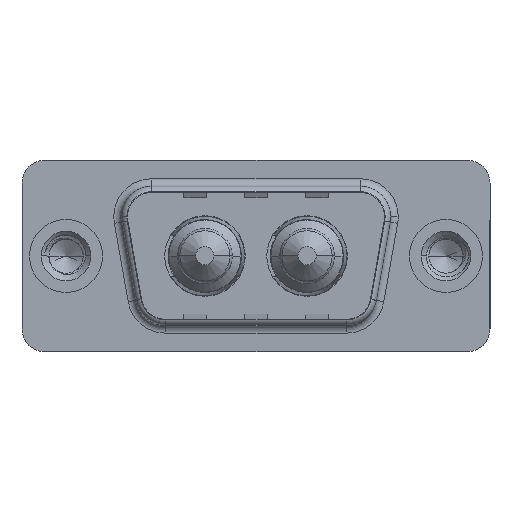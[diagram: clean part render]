
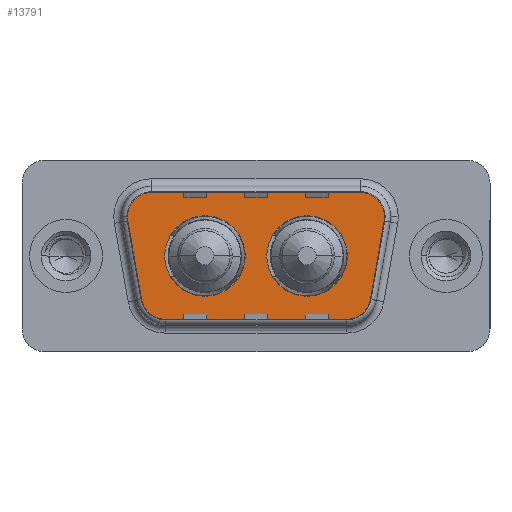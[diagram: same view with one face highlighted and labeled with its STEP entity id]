
A CAD part, top view. The second image highlights one B-rep face of the part: STEP entity #13791.
In plain terms, the highlighted planar face has unit normal (0, 0, 1).
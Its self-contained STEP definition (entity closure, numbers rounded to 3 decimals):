
#333 = DIRECTION ( 'NONE',  ( 1., 0., 0. ) ) ;
#508 = EDGE_CURVE ( 'NONE', #4184, #7738, #15613, .T. ) ;
#585 = EDGE_CURVE ( 'NONE', #8998, #4009, #1623, .T. ) ;
#634 = ORIENTED_EDGE ( 'NONE', *, *, #4315, .F. ) ;
#1050 = VERTEX_POINT ( 'NONE', #10100 ) ;
#1607 = CIRCLE ( 'NONE', #13384, 2. ) ;
#1623 = LINE ( 'NONE', #12045, #7820 ) ;
#1780 = EDGE_CURVE ( 'NONE', #1050, #6026, #15411, .T. ) ;
#2015 = VECTOR ( 'NONE', #2477, 1000. ) ;
#2201 = VECTOR ( 'NONE', #15428, 1000. ) ;
#2207 = EDGE_CURVE ( 'NONE', #7170, #6162, #10963, .T. ) ;
#2226 = EDGE_CURVE ( 'NONE', #14384, #4184, #1607, .T. ) ;
#2374 = CARTESIAN_POINT ( 'NONE',  ( 19.564, 2.9, 0. ) ) ;
#2419 = EDGE_CURVE ( 'NONE', #6162, #11359, #12398, .T. ) ;
#2477 = DIRECTION ( 'NONE',  ( -1., 0., 0. ) ) ;
#2572 = AXIS2_PLACEMENT_3D ( 'NONE', #5162, #15972, #12566 ) ;
#2642 = ORIENTED_EDGE ( 'NONE', *, *, #10940, .F. ) ;
#2664 = PLANE ( 'NONE',  #12718 ) ;
#2743 = CARTESIAN_POINT ( 'NONE',  ( 5.436, 4.9, 0. ) ) ;
#2938 = CARTESIAN_POINT ( 'NONE',  ( 5.436, 2.9, 0. ) ) ;
#3578 = CARTESIAN_POINT ( 'NONE',  ( 6.459, -4.9, 0. ) ) ;
#3645 = ORIENTED_EDGE ( 'NONE', *, *, #508, .T. ) ;
#3659 = DIRECTION ( 'NONE',  ( -1., 0., 0. ) ) ;
#3669 = AXIS2_PLACEMENT_3D ( 'NONE', #6401, #7185, #7149 ) ;
#3934 = DIRECTION ( 'NONE',  ( 1., 0., 0. ) ) ;
#3965 = VERTEX_POINT ( 'NONE', #11274 ) ;
#4009 = VERTEX_POINT ( 'NONE', #14877 ) ;
#4057 = CIRCLE ( 'NONE', #5607, 2. ) ;
#4184 = VERTEX_POINT ( 'NONE', #5513 ) ;
#4235 = DIRECTION ( 'NONE',  ( 1., 0., 0. ) ) ;
#4248 = AXIS2_PLACEMENT_3D ( 'NONE', #2374, #11283, #3659 ) ;
#4315 = EDGE_CURVE ( 'NONE', #15826, #9567, #7523, .T. ) ;
#4440 = CARTESIAN_POINT ( 'NONE',  ( 19.564, 2.9, 0. ) ) ;
#4667 = EDGE_CURVE ( 'NONE', #6026, #1050, #10710, .T. ) ;
#4704 = LINE ( 'NONE', #3578, #10680 ) ;
#4769 = ORIENTED_EDGE ( 'NONE', *, *, #2419, .T. ) ;
#4831 = CARTESIAN_POINT ( 'NONE',  ( 13.21, 0., 0. ) ) ;
#4928 = CARTESIAN_POINT ( 'NONE',  ( 3.466, 2.553, 0. ) ) ;
#4992 = DIRECTION ( 'NONE',  ( 0., 0., 1. ) ) ;
#5029 = CARTESIAN_POINT ( 'NONE',  ( 11.79, 0., 0. ) ) ;
#5162 = CARTESIAN_POINT ( 'NONE',  ( 15.86, 0., 0. ) ) ;
#5513 = CARTESIAN_POINT ( 'NONE',  ( 19.564, 4.9, 0. ) ) ;
#5607 = AXIS2_PLACEMENT_3D ( 'NONE', #12652, #4992, #13917 ) ;
#5917 = EDGE_CURVE ( 'NONE', #3965, #7170, #4704, .T. ) ;
#6026 = VERTEX_POINT ( 'NONE', #4831 ) ;
#6162 = VERTEX_POINT ( 'NONE', #15930 ) ;
#6401 = CARTESIAN_POINT ( 'NONE',  ( 15.86, 0., 0. ) ) ;
#6519 = DIRECTION ( 'NONE',  ( 1., 0., 0. ) ) ;
#6586 = ORIENTED_EDGE ( 'NONE', *, *, #8047, .T. ) ;
#7071 = DIRECTION ( 'NONE',  ( 0., 0., 1. ) ) ;
#7118 = EDGE_LOOP ( 'NONE', ( #2642, #634 ) ) ;
#7149 = DIRECTION ( 'NONE',  ( 1., 0., 0. ) ) ;
#7170 = VERTEX_POINT ( 'NONE', #13029 ) ;
#7185 = DIRECTION ( 'NONE',  ( 0., 0., 1. ) ) ;
#7472 = CARTESIAN_POINT ( 'NONE',  ( 5.436, 4.9, 0. ) ) ;
#7509 = EDGE_CURVE ( 'NONE', #4009, #3965, #4057, .T. ) ;
#7523 = CIRCLE ( 'NONE', #12857, 2.65 ) ;
#7738 = VERTEX_POINT ( 'NONE', #2743 ) ;
#7820 = VECTOR ( 'NONE', #11734, 1000. ) ;
#7966 = DIRECTION ( 'NONE',  ( 0., 0., 1. ) ) ;
#8047 = EDGE_CURVE ( 'NONE', #7738, #8998, #8244, .T. ) ;
#8189 = ORIENTED_EDGE ( 'NONE', *, *, #2226, .T. ) ;
#8205 = EDGE_LOOP ( 'NONE', ( #10204, #4769, #11759, #8189, #3645, #6586, #12038, #10561, #8634 ) ) ;
#8244 = CIRCLE ( 'NONE', #14396, 2. ) ;
#8346 = DIRECTION ( 'NONE',  ( 0., 0., 1. ) ) ;
#8549 = FACE_BOUND ( 'NONE', #7118, .T. ) ;
#8634 = ORIENTED_EDGE ( 'NONE', *, *, #5917, .T. ) ;
#8866 = AXIS2_PLACEMENT_3D ( 'NONE', #15650, #7966, #333 ) ;
#8954 = FACE_OUTER_BOUND ( 'NONE', #8205, .T. ) ;
#8998 = VERTEX_POINT ( 'NONE', #4928 ) ;
#9567 = VERTEX_POINT ( 'NONE', #5029 ) ;
#9751 = CARTESIAN_POINT ( 'NONE',  ( 18.541, -2.9, 0. ) ) ;
#9790 = DIRECTION ( 'NONE',  ( 0., 0., 1. ) ) ;
#9984 = CARTESIAN_POINT ( 'NONE',  ( 21.534, 2.553, 0. ) ) ;
#9985 = AXIS2_PLACEMENT_3D ( 'NONE', #9751, #9790, #14906 ) ;
#10100 = CARTESIAN_POINT ( 'NONE',  ( 18.51, 0., 0. ) ) ;
#10204 = ORIENTED_EDGE ( 'NONE', *, *, #2207, .T. ) ;
#10561 = ORIENTED_EDGE ( 'NONE', *, *, #7509, .T. ) ;
#10680 = VECTOR ( 'NONE', #6519, 1000. ) ;
#10710 = CIRCLE ( 'NONE', #3669, 2.65 ) ;
#10940 = EDGE_CURVE ( 'NONE', #9567, #15826, #13869, .T. ) ;
#10963 = CIRCLE ( 'NONE', #9985, 2. ) ;
#11006 = CARTESIAN_POINT ( 'NONE',  ( 9.14, 0., 0. ) ) ;
#11147 = EDGE_CURVE ( 'NONE', #11359, #14384, #11457, .T. ) ;
#11274 = CARTESIAN_POINT ( 'NONE',  ( 6.459, -4.9, 0. ) ) ;
#11283 = DIRECTION ( 'NONE',  ( 0., 0., 1. ) ) ;
#11359 = VERTEX_POINT ( 'NONE', #12903 ) ;
#11457 = CIRCLE ( 'NONE', #4248, 2. ) ;
#11578 = DIRECTION ( 'NONE',  ( 0., 0., 1. ) ) ;
#11734 = DIRECTION ( 'NONE',  ( 0.174, -0.985, 0. ) ) ;
#11759 = ORIENTED_EDGE ( 'NONE', *, *, #11147, .T. ) ;
#11881 = DIRECTION ( 'NONE',  ( 0., 0., 1. ) ) ;
#12027 = ORIENTED_EDGE ( 'NONE', *, *, #1780, .F. ) ;
#12038 = ORIENTED_EDGE ( 'NONE', *, *, #585, .T. ) ;
#12045 = CARTESIAN_POINT ( 'NONE',  ( 3.466, 2.553, 0. ) ) ;
#12050 = DIRECTION ( 'NONE',  ( -1., 0., 0. ) ) ;
#12398 = LINE ( 'NONE', #9984, #2201 ) ;
#12405 = CARTESIAN_POINT ( 'NONE',  ( 21.564, 2.9, 0. ) ) ;
#12429 = ORIENTED_EDGE ( 'NONE', *, *, #4667, .F. ) ;
#12566 = DIRECTION ( 'NONE',  ( 1., 0., 0. ) ) ;
#12652 = CARTESIAN_POINT ( 'NONE',  ( 6.459, -2.9, 0. ) ) ;
#12718 = AXIS2_PLACEMENT_3D ( 'NONE', #12822, #11578, #3934 ) ;
#12822 = CARTESIAN_POINT ( 'NONE',  ( 18.541, -2.9, 0. ) ) ;
#12857 = AXIS2_PLACEMENT_3D ( 'NONE', #11006, #7071, #13764 ) ;
#12903 = CARTESIAN_POINT ( 'NONE',  ( 21.534, 2.553, 0. ) ) ;
#13029 = CARTESIAN_POINT ( 'NONE',  ( 18.541, -4.9, 0. ) ) ;
#13384 = AXIS2_PLACEMENT_3D ( 'NONE', #4440, #8346, #12050 ) ;
#13749 = CARTESIAN_POINT ( 'NONE',  ( 6.49, 0., 0. ) ) ;
#13764 = DIRECTION ( 'NONE',  ( 1., 0., 0. ) ) ;
#13791 = ADVANCED_FACE ( 'NONE', ( #15355, #8549, #8954 ), #2664, .T. ) ;
#13869 = CIRCLE ( 'NONE', #8866, 2.65 ) ;
#13917 = DIRECTION ( 'NONE',  ( -1., 0., 0. ) ) ;
#14384 = VERTEX_POINT ( 'NONE', #12405 ) ;
#14396 = AXIS2_PLACEMENT_3D ( 'NONE', #2938, #11881, #4235 ) ;
#14877 = CARTESIAN_POINT ( 'NONE',  ( 4.489, -3.247, 0. ) ) ;
#14906 = DIRECTION ( 'NONE',  ( 1., 0., 0. ) ) ;
#15355 = FACE_BOUND ( 'NONE', #15555, .T. ) ;
#15411 = CIRCLE ( 'NONE', #2572, 2.65 ) ;
#15428 = DIRECTION ( 'NONE',  ( 0.174, 0.985, 0. ) ) ;
#15555 = EDGE_LOOP ( 'NONE', ( #12027, #12429 ) ) ;
#15613 = LINE ( 'NONE', #7472, #2015 ) ;
#15650 = CARTESIAN_POINT ( 'NONE',  ( 9.14, 0., 0. ) ) ;
#15826 = VERTEX_POINT ( 'NONE', #13749 ) ;
#15930 = CARTESIAN_POINT ( 'NONE',  ( 20.511, -3.247, 0. ) ) ;
#15972 = DIRECTION ( 'NONE',  ( 0., 0., 1. ) ) ;
